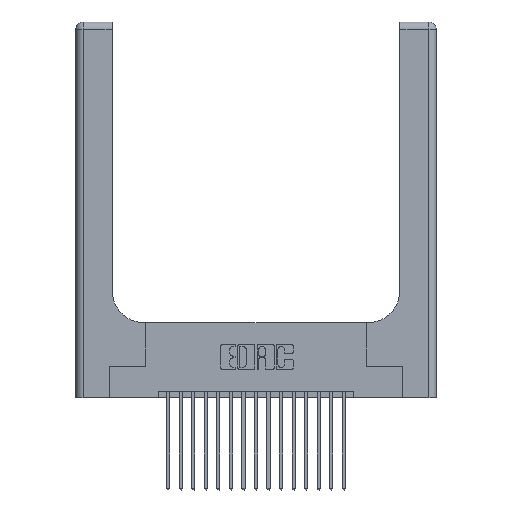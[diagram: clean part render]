
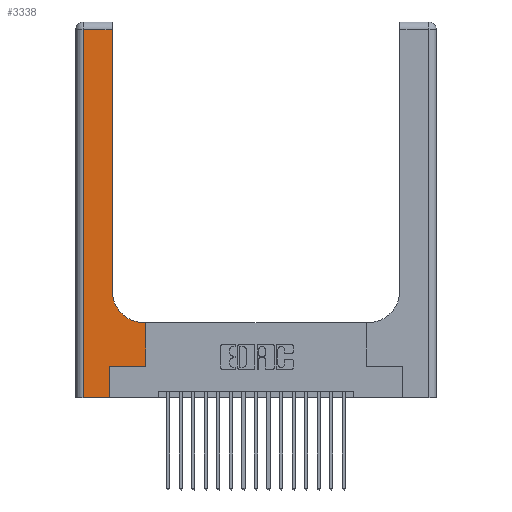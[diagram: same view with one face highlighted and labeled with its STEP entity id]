
A CAD part, top view. The second image highlights one B-rep face of the part: STEP entity #3338.
In plain terms, the highlighted planar face has unit normal (0, 0, 1).
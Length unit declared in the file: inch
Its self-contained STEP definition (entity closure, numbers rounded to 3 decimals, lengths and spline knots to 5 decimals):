
#144 = EDGE_CURVE ( 'NONE', #1641, #15690, #3119, .T. ) ;
#643 = DIRECTION ( 'NONE',  ( 0., -1., 0. ) ) ;
#711 = CARTESIAN_POINT ( 'NONE',  ( 0.5585, 0.25, 0.37 ) ) ;
#877 = VECTOR ( 'NONE', #18327, 39.37008 ) ;
#990 = EDGE_CURVE ( 'NONE', #1372, #14167, #14520, .T. ) ;
#1372 = VERTEX_POINT ( 'NONE', #711 ) ;
#1641 = VERTEX_POINT ( 'NONE', #20325 ) ;
#1788 = CARTESIAN_POINT ( 'NONE',  ( 0.269, 0.25, 0.37 ) ) ;
#1929 = EDGE_LOOP ( 'NONE', ( #10128, #10147, #10500, #10677, #10900, #11175, #11409, #11642, #11681 ) ) ;
#2123 = CARTESIAN_POINT ( 'NONE',  ( 0., 3., 0.37 ) ) ;
#2406 = CARTESIAN_POINT ( 'NONE',  ( 0.2915, 0.6, 0.37 ) ) ;
#3119 = LINE ( 'NONE', #13399, #19483 ) ;
#3338 = ADVANCED_FACE ( 'NONE', ( #15699 ), #13272, .F. ) ;
#3428 = CARTESIAN_POINT ( 'NONE',  ( 0.2915, 3., 0.37 ) ) ;
#3785 = VERTEX_POINT ( 'NONE', #6342 ) ;
#5378 = DIRECTION ( 'NONE',  ( -1., 0., 0. ) ) ;
#5602 = VECTOR ( 'NONE', #8155, 39.37008 ) ;
#5666 = CARTESIAN_POINT ( 'NONE',  ( 0.2915, 0.85, 0.37 ) ) ;
#6149 = EDGE_CURVE ( 'NONE', #7869, #10262, #14957, .T. ) ;
#6342 = CARTESIAN_POINT ( 'NONE',  ( 0.2915, 2.94, 0.37 ) ) ;
#7026 = VECTOR ( 'NONE', #15829, 39.37008 ) ;
#7713 = VERTEX_POINT ( 'NONE', #9854 ) ;
#7869 = VERTEX_POINT ( 'NONE', #16835 ) ;
#8155 = DIRECTION ( 'NONE',  ( 0., 1., 0. ) ) ;
#8197 = CARTESIAN_POINT ( 'NONE',  ( 0.5585, 0.25, 0.37 ) ) ;
#8276 = AXIS2_PLACEMENT_3D ( 'NONE', #2123, #14862, #5378 ) ;
#8285 = DIRECTION ( 'NONE',  ( 1., 0., 0. ) ) ;
#8546 = DIRECTION ( 'NONE',  ( 0., 0., -1. ) ) ;
#8668 = CARTESIAN_POINT ( 'NONE',  ( 0.269, 0.25, 0.37 ) ) ;
#9366 = VECTOR ( 'NONE', #18666, 39.37008 ) ;
#9793 = EDGE_CURVE ( 'NONE', #3785, #1641, #13590, .T. ) ;
#9854 = CARTESIAN_POINT ( 'NONE',  ( 0.5415, 0.6, 0.37 ) ) ;
#10128 = ORIENTED_EDGE ( 'NONE', *, *, #15386, .T. ) ;
#10147 = ORIENTED_EDGE ( 'NONE', *, *, #9793, .T. ) ;
#10262 = VERTEX_POINT ( 'NONE', #8668 ) ;
#10304 = VECTOR ( 'NONE', #8285, 39.37008 ) ;
#10500 = ORIENTED_EDGE ( 'NONE', *, *, #144, .T. ) ;
#10677 = ORIENTED_EDGE ( 'NONE', *, *, #13449, .T. ) ;
#10783 = CIRCLE ( 'NONE', #18092, 0.25 ) ;
#10785 = CARTESIAN_POINT ( 'NONE',  ( 0., 0., 0.37 ) ) ;
#10900 = ORIENTED_EDGE ( 'NONE', *, *, #6149, .T. ) ;
#10908 = VECTOR ( 'NONE', #14532, 39.37008 ) ;
#11175 = ORIENTED_EDGE ( 'NONE', *, *, #17805, .T. ) ;
#11409 = ORIENTED_EDGE ( 'NONE', *, *, #990, .T. ) ;
#11515 = EDGE_CURVE ( 'NONE', #7713, #12899, #10783, .T. ) ;
#11642 = ORIENTED_EDGE ( 'NONE', *, *, #19059, .T. ) ;
#11681 = ORIENTED_EDGE ( 'NONE', *, *, #11515, .T. ) ;
#11964 = VECTOR ( 'NONE', #13927, 39.37008 ) ;
#12899 = VERTEX_POINT ( 'NONE', #5666 ) ;
#13272 = PLANE ( 'NONE',  #8276 ) ;
#13399 = CARTESIAN_POINT ( 'NONE',  ( 0.06, 3., 0.37 ) ) ;
#13449 = EDGE_CURVE ( 'NONE', #15690, #7869, #15208, .T. ) ;
#13590 = LINE ( 'NONE', #13896, #9366 ) ;
#13896 = CARTESIAN_POINT ( 'NONE',  ( 0., 2.94, 0.37 ) ) ;
#13927 = DIRECTION ( 'NONE',  ( 1., 0., 0. ) ) ;
#14167 = VERTEX_POINT ( 'NONE', #14247 ) ;
#14247 = CARTESIAN_POINT ( 'NONE',  ( 0.5585, 0.6, 0.37 ) ) ;
#14520 = LINE ( 'NONE', #8197, #5602 ) ;
#14532 = DIRECTION ( 'NONE',  ( 0., 1., 0. ) ) ;
#14634 = LINE ( 'NONE', #3428, #10908 ) ;
#14862 = DIRECTION ( 'NONE',  ( 0., 0., -1. ) ) ;
#14957 = LINE ( 'NONE', #18938, #7026 ) ;
#15041 = LINE ( 'NONE', #1788, #10304 ) ;
#15208 = LINE ( 'NONE', #10785, #11964 ) ;
#15386 = EDGE_CURVE ( 'NONE', #12899, #3785, #14634, .T. ) ;
#15417 = CARTESIAN_POINT ( 'NONE',  ( 0.06, 0., 0.37 ) ) ;
#15690 = VERTEX_POINT ( 'NONE', #15417 ) ;
#15699 = FACE_OUTER_BOUND ( 'NONE', #1929, .T. ) ;
#15829 = DIRECTION ( 'NONE',  ( 0., 1., 0. ) ) ;
#16835 = CARTESIAN_POINT ( 'NONE',  ( 0.269, 0., 0.37 ) ) ;
#17786 = LINE ( 'NONE', #2406, #877 ) ;
#17805 = EDGE_CURVE ( 'NONE', #10262, #1372, #15041, .T. ) ;
#18018 = CARTESIAN_POINT ( 'NONE',  ( 0.5415, 0.85, 0.37 ) ) ;
#18092 = AXIS2_PLACEMENT_3D ( 'NONE', #18018, #8546, #19623 ) ;
#18327 = DIRECTION ( 'NONE',  ( -1., 0., 0. ) ) ;
#18666 = DIRECTION ( 'NONE',  ( -1., 0., 0. ) ) ;
#18938 = CARTESIAN_POINT ( 'NONE',  ( 0.269, 0., 0.37 ) ) ;
#19059 = EDGE_CURVE ( 'NONE', #14167, #7713, #17786, .T. ) ;
#19483 = VECTOR ( 'NONE', #643, 39.37008 ) ;
#19623 = DIRECTION ( 'NONE',  ( 1., 0., 0. ) ) ;
#20325 = CARTESIAN_POINT ( 'NONE',  ( 0.06, 2.94, 0.37 ) ) ;
